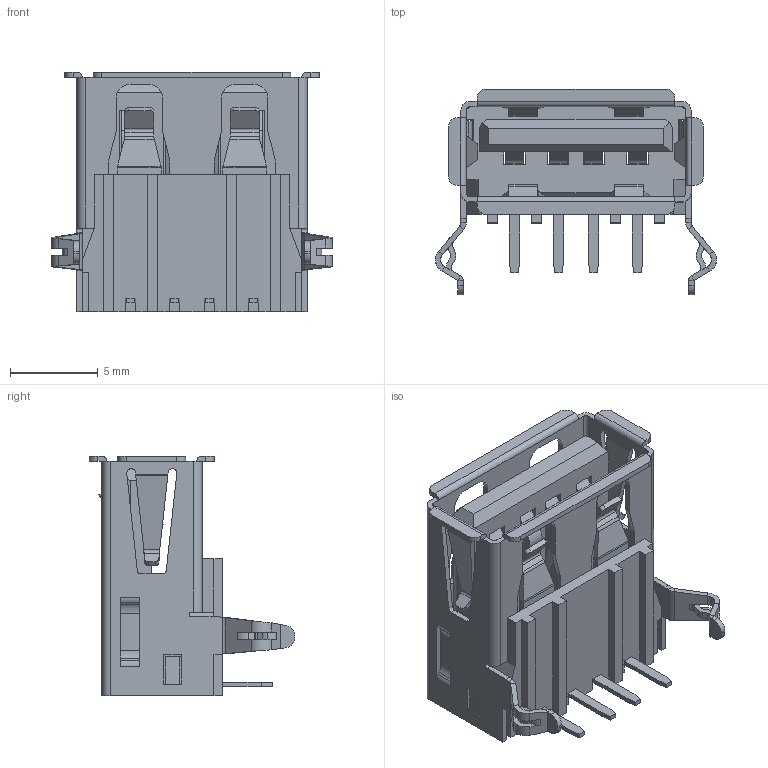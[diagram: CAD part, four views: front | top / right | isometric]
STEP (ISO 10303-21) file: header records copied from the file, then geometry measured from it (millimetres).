
FILE_DESCRIPTION (( 'STEP AP214' ), '1' );
FILE_NAME ('690A104-123-411.STEP', '2021-01-13T21:12:24', ( '' ), ( '' ), 'SwSTEP 2.0', 'SolidWorks 2020', '' );
FILE_SCHEMA (( 'AUTOMOTIVE_DESIGN' ));
Length unit declared in the file: millimetre
Products named in the file (4): Insulator 690A104-X23-4XX_Black; Shell 690A104-X23-4XX; 690A104-123-411; Contact 690A104-X23-4XX
Assembly tree (6 placements, depth 2):
  690A104-123-411
    Insulator 690A104-X23-4XX_Black
    Contact 690A104-X23-4XX  x4
    Shell 690A104-X23-4XX
Bounding box: 16 x 11.7 x 13.65 mm (x, y, z)
Volume: 556.6 mm3; surface area: 2007.5 mm2
Topology: 6 solids, 6 shells, 826 faces, 2303 edges, 1468 vertices
Faces by surface type: plane 606, cylinder 184, bspline 36
Entity records: 22161 total; most frequent: CARTESIAN_POINT 5078, ORIENTED_EDGE 3688, DIRECTION 3296, EDGE_CURVE 1844, LINE 1474, VECTOR 1474, VERTEX_POINT 1162, AXIS2_PLACEMENT_3D 911
